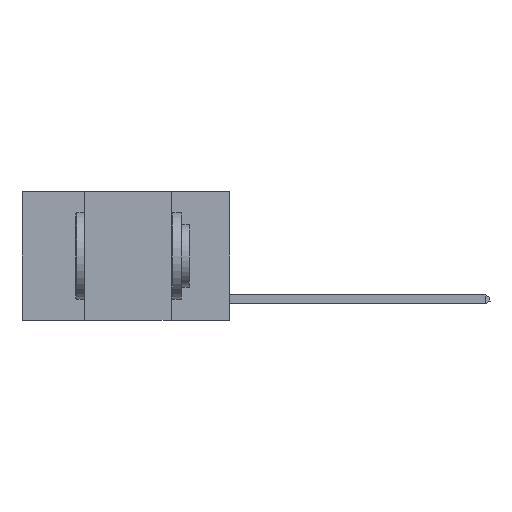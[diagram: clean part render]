
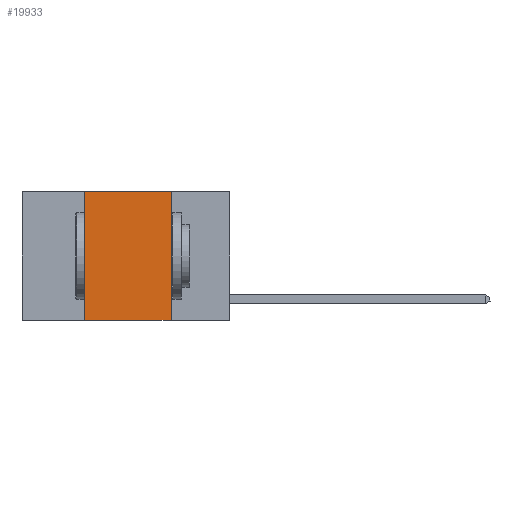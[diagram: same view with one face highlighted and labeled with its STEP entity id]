
A CAD part, left-side view. The second image highlights one B-rep face of the part: STEP entity #19933.
In plain terms, the highlighted planar face has unit normal (-1, 0, 0).
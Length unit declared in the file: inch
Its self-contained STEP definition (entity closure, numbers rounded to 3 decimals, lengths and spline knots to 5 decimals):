
#81 = EDGE_CURVE ( 'NONE', #2323, #21861, #19744, .T. ) ;
#1114 = FACE_OUTER_BOUND ( 'NONE', #3643, .T. ) ;
#1446 = DIRECTION ( 'NONE',  ( 1., 0., 0. ) ) ;
#1455 = CARTESIAN_POINT ( 'NONE',  ( 0., 0.42, 0. ) ) ;
#2323 = VERTEX_POINT ( 'NONE', #16165 ) ;
#3643 = EDGE_LOOP ( 'NONE', ( #21108, #22419, #23068, #7509 ) ) ;
#4916 = CARTESIAN_POINT ( 'NONE',  ( 0., 0.17, 0. ) ) ;
#7509 = ORIENTED_EDGE ( 'NONE', *, *, #81, .T. ) ;
#8427 = VECTOR ( 'NONE', #11647, 39.37008 ) ;
#8688 = CARTESIAN_POINT ( 'NONE',  ( 0., 0.42, 0. ) ) ;
#10010 = EDGE_CURVE ( 'NONE', #2323, #26242, #24007, .T. ) ;
#11423 = EDGE_CURVE ( 'NONE', #18847, #21861, #21314, .T. ) ;
#11647 = DIRECTION ( 'NONE',  ( 0., -1., 0. ) ) ;
#12921 = VECTOR ( 'NONE', #19001, 39.37008 ) ;
#14144 = CARTESIAN_POINT ( 'NONE',  ( 0., 0.6, 0. ) ) ;
#14201 = EDGE_CURVE ( 'NONE', #26242, #18847, #24146, .T. ) ;
#14886 = CARTESIAN_POINT ( 'NONE',  ( 0., 0.6, 0. ) ) ;
#16165 = CARTESIAN_POINT ( 'NONE',  ( 0., 0.42, -0.37 ) ) ;
#16275 = DIRECTION ( 'NONE',  ( 0., 0., -1. ) ) ;
#17015 = AXIS2_PLACEMENT_3D ( 'NONE', #14144, #1446, #16275 ) ;
#18410 = VECTOR ( 'NONE', #23493, 39.37008 ) ;
#18847 = VERTEX_POINT ( 'NONE', #23334 ) ;
#19001 = DIRECTION ( 'NONE',  ( 0., -1., 0. ) ) ;
#19209 = CARTESIAN_POINT ( 'NONE',  ( 0., 0.17, -0.37 ) ) ;
#19744 = LINE ( 'NONE', #21220, #8427 ) ;
#19933 = ADVANCED_FACE ( 'NONE', ( #1114 ), #26754, .F. ) ;
#21108 = ORIENTED_EDGE ( 'NONE', *, *, #11423, .F. ) ;
#21220 = CARTESIAN_POINT ( 'NONE',  ( 0., 0.6, -0.37 ) ) ;
#21314 = LINE ( 'NONE', #4916, #26206 ) ;
#21861 = VERTEX_POINT ( 'NONE', #19209 ) ;
#22419 = ORIENTED_EDGE ( 'NONE', *, *, #14201, .F. ) ;
#23068 = ORIENTED_EDGE ( 'NONE', *, *, #10010, .F. ) ;
#23334 = CARTESIAN_POINT ( 'NONE',  ( 0., 0.17, 0. ) ) ;
#23493 = DIRECTION ( 'NONE',  ( 0., 0., 1. ) ) ;
#24007 = LINE ( 'NONE', #8688, #18410 ) ;
#24146 = LINE ( 'NONE', #14886, #12921 ) ;
#26054 = DIRECTION ( 'NONE',  ( 0., 0., -1. ) ) ;
#26206 = VECTOR ( 'NONE', #26054, 39.37008 ) ;
#26242 = VERTEX_POINT ( 'NONE', #1455 ) ;
#26754 = PLANE ( 'NONE',  #17015 ) ;
